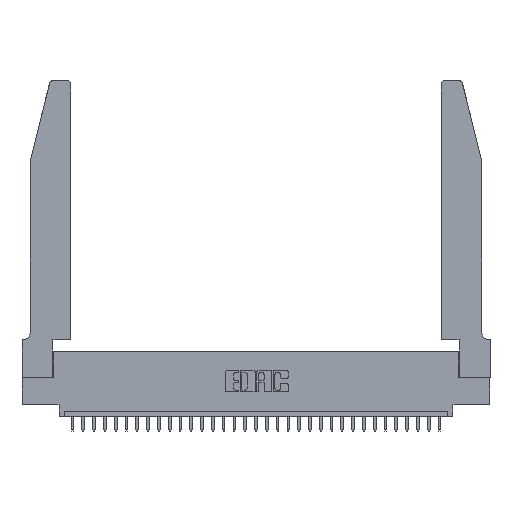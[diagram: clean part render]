
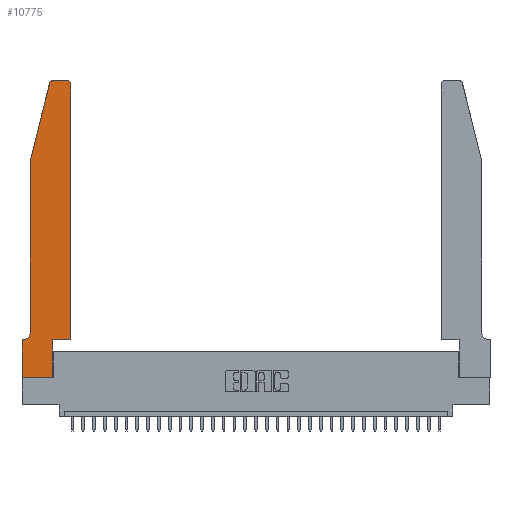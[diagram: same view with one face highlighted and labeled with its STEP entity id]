
A CAD part, top view. The second image highlights one B-rep face of the part: STEP entity #10775.
In plain terms, the highlighted planar face has unit normal (0, 0, 1).
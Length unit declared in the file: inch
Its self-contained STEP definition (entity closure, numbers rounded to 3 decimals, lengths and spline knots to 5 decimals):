
#240 = CARTESIAN_POINT ( 'NONE',  ( 0.4205, 2.72, 0.37 ) ) ;
#623 = VECTOR ( 'NONE', #9266, 39.37008 ) ;
#679 = ORIENTED_EDGE ( 'NONE', *, *, #16716, .T. ) ;
#1439 = CARTESIAN_POINT ( 'NONE',  ( 0.4505, 2.72, 0.37 ) ) ;
#1793 = CARTESIAN_POINT ( 'NONE',  ( 0.2865, 0., 0.37 ) ) ;
#2167 = LINE ( 'NONE', #10430, #25486 ) ;
#2177 = CIRCLE ( 'NONE', #19346, 0.07 ) ;
#2234 = PLANE ( 'NONE',  #19637 ) ;
#2331 = DIRECTION ( 'NONE',  ( 0., 0., 1. ) ) ;
#2535 = VECTOR ( 'NONE', #6171, 39.37008 ) ;
#2727 = DIRECTION ( 'NONE',  ( 0., 0., 1. ) ) ;
#3883 = ORIENTED_EDGE ( 'NONE', *, *, #8492, .T. ) ;
#3891 = LINE ( 'NONE', #27570, #7743 ) ;
#4243 = VERTEX_POINT ( 'NONE', #7060 ) ;
#4352 = LINE ( 'NONE', #8504, #17200 ) ;
#4415 = LINE ( 'NONE', #30306, #8326 ) ;
#4487 = CARTESIAN_POINT ( 'NONE',  ( 0.284, 2.75, 0.37 ) ) ;
#5235 = DIRECTION ( 'NONE',  ( 1., 0., 0. ) ) ;
#5300 = DIRECTION ( 'NONE',  ( 0., -1., 0. ) ) ;
#5750 = LINE ( 'NONE', #9381, #26382 ) ;
#6125 = CARTESIAN_POINT ( 'NONE',  ( 0., 0.35, 0.37 ) ) ;
#6171 = DIRECTION ( 'NONE',  ( 1., 0., 0. ) ) ;
#6735 = ORIENTED_EDGE ( 'NONE', *, *, #15269, .T. ) ;
#7060 = CARTESIAN_POINT ( 'NONE',  ( 0.4505, 0.35, 0.37 ) ) ;
#7451 = ORIENTED_EDGE ( 'NONE', *, *, #8089, .T. ) ;
#7743 = VECTOR ( 'NONE', #7985, 39.37008 ) ;
#7943 = DIRECTION ( 'NONE',  ( 0., -1., 0. ) ) ;
#7962 = VERTEX_POINT ( 'NONE', #10109 ) ;
#7985 = DIRECTION ( 'NONE',  ( -1., 0., 0. ) ) ;
#8089 = EDGE_CURVE ( 'NONE', #11727, #10027, #4352, .T. ) ;
#8212 = DIRECTION ( 'NONE',  ( 0., 0., -1. ) ) ;
#8326 = VECTOR ( 'NONE', #17617, 39.37008 ) ;
#8492 = EDGE_CURVE ( 'NONE', #19123, #4243, #9518, .T. ) ;
#8504 = CARTESIAN_POINT ( 'NONE',  ( 0.0755, 2., 0.37 ) ) ;
#9266 = DIRECTION ( 'NONE',  ( 0., 1., 0. ) ) ;
#9381 = CARTESIAN_POINT ( 'NONE',  ( 0.2865, 0.35, 0.37 ) ) ;
#9518 = LINE ( 'NONE', #30940, #2535 ) ;
#9547 = CARTESIAN_POINT ( 'NONE',  ( 0.284, 2.72, 0.37 ) ) ;
#10027 = VERTEX_POINT ( 'NONE', #22442 ) ;
#10109 = CARTESIAN_POINT ( 'NONE',  ( 0.0055, 0.35, 0.37 ) ) ;
#10288 = EDGE_LOOP ( 'NONE', ( #25359, #13772, #23497, #7451, #28519, #15678, #6735, #679, #15769, #3883, #28591, #28400 ) ) ;
#10430 = CARTESIAN_POINT ( 'NONE',  ( 0., 0., 0.37 ) ) ;
#10566 = CARTESIAN_POINT ( 'NONE',  ( 0.2865, 0.35, 0.37 ) ) ;
#10775 = ADVANCED_FACE ( 'NONE', ( #23770 ), #2234, .T. ) ;
#11593 = AXIS2_PLACEMENT_3D ( 'NONE', #240, #2727, #5235 ) ;
#11727 = VERTEX_POINT ( 'NONE', #25928 ) ;
#12066 = DIRECTION ( 'NONE',  ( 1., 0., 0. ) ) ;
#12203 = VECTOR ( 'NONE', #26372, 39.37008 ) ;
#12332 = EDGE_CURVE ( 'NONE', #15940, #11727, #15916, .T. ) ;
#13433 = EDGE_CURVE ( 'NONE', #10027, #7962, #2177, .T. ) ;
#13578 = CARTESIAN_POINT ( 'NONE',  ( 0.0055, 0.42, 0.37 ) ) ;
#13636 = CIRCLE ( 'NONE', #19750, 0.03 ) ;
#13772 = ORIENTED_EDGE ( 'NONE', *, *, #23949, .T. ) ;
#14509 = EDGE_CURVE ( 'NONE', #20005, #19123, #5750, .T. ) ;
#14687 = VERTEX_POINT ( 'NONE', #6125 ) ;
#15269 = EDGE_CURVE ( 'NONE', #14687, #28038, #2167, .T. ) ;
#15318 = CARTESIAN_POINT ( 'NONE',  ( 0.0755, 2., 0.37 ) ) ;
#15678 = ORIENTED_EDGE ( 'NONE', *, *, #24137, .T. ) ;
#15769 = ORIENTED_EDGE ( 'NONE', *, *, #14509, .T. ) ;
#15916 = LINE ( 'NONE', #15318, #21728 ) ;
#15940 = VERTEX_POINT ( 'NONE', #30138 ) ;
#16716 = EDGE_CURVE ( 'NONE', #28038, #20005, #18808, .T. ) ;
#17068 = CIRCLE ( 'NONE', #11593, 0.03 ) ;
#17200 = VECTOR ( 'NONE', #5300, 39.37008 ) ;
#17617 = DIRECTION ( 'NONE',  ( -1., 0., 0. ) ) ;
#18340 = DIRECTION ( 'NONE',  ( -1., 0., 0. ) ) ;
#18510 = LINE ( 'NONE', #26485, #623 ) ;
#18808 = LINE ( 'NONE', #31435, #12203 ) ;
#19123 = VERTEX_POINT ( 'NONE', #10566 ) ;
#19346 = AXIS2_PLACEMENT_3D ( 'NONE', #13578, #8212, #18340 ) ;
#19637 = AXIS2_PLACEMENT_3D ( 'NONE', #32131, #2331, #24763 ) ;
#19750 = AXIS2_PLACEMENT_3D ( 'NONE', #9547, #26967, #12066 ) ;
#19926 = EDGE_CURVE ( 'NONE', #26580, #24347, #17068, .T. ) ;
#20005 = VERTEX_POINT ( 'NONE', #1793 ) ;
#21728 = VECTOR ( 'NONE', #29626, 39.37008 ) ;
#21796 = EDGE_CURVE ( 'NONE', #24347, #30751, #4415, .T. ) ;
#22442 = CARTESIAN_POINT ( 'NONE',  ( 0.0755, 0.42, 0.37 ) ) ;
#22602 = DIRECTION ( 'NONE',  ( 0., 1., 0. ) ) ;
#23222 = CARTESIAN_POINT ( 'NONE',  ( 0.4205, 2.75, 0.37 ) ) ;
#23497 = ORIENTED_EDGE ( 'NONE', *, *, #12332, .T. ) ;
#23770 = FACE_OUTER_BOUND ( 'NONE', #10288, .T. ) ;
#23949 = EDGE_CURVE ( 'NONE', #30751, #15940, #13636, .T. ) ;
#24137 = EDGE_CURVE ( 'NONE', #7962, #14687, #3891, .T. ) ;
#24347 = VERTEX_POINT ( 'NONE', #23222 ) ;
#24763 = DIRECTION ( 'NONE',  ( 1., 0., 0. ) ) ;
#25359 = ORIENTED_EDGE ( 'NONE', *, *, #21796, .T. ) ;
#25486 = VECTOR ( 'NONE', #7943, 39.37008 ) ;
#25928 = CARTESIAN_POINT ( 'NONE',  ( 0.0755, 2., 0.37 ) ) ;
#26372 = DIRECTION ( 'NONE',  ( 1., 0., 0. ) ) ;
#26382 = VECTOR ( 'NONE', #22602, 39.37008 ) ;
#26485 = CARTESIAN_POINT ( 'NONE',  ( 0.4505, 0.35, 0.37 ) ) ;
#26580 = VERTEX_POINT ( 'NONE', #1439 ) ;
#26967 = DIRECTION ( 'NONE',  ( 0., 0., 1. ) ) ;
#27106 = CARTESIAN_POINT ( 'NONE',  ( 0., 0., 0.37 ) ) ;
#27570 = CARTESIAN_POINT ( 'NONE',  ( 0.0755, 0.35, 0.37 ) ) ;
#27884 = EDGE_CURVE ( 'NONE', #4243, #26580, #18510, .T. ) ;
#28038 = VERTEX_POINT ( 'NONE', #27106 ) ;
#28400 = ORIENTED_EDGE ( 'NONE', *, *, #19926, .T. ) ;
#28519 = ORIENTED_EDGE ( 'NONE', *, *, #13433, .T. ) ;
#28591 = ORIENTED_EDGE ( 'NONE', *, *, #27884, .T. ) ;
#29626 = DIRECTION ( 'NONE',  ( -0.239, -0.971, 0. ) ) ;
#30138 = CARTESIAN_POINT ( 'NONE',  ( 0.25487, 2.72718, 0.37 ) ) ;
#30306 = CARTESIAN_POINT ( 'NONE',  ( 0.2605, 2.75, 0.37 ) ) ;
#30751 = VERTEX_POINT ( 'NONE', #4487 ) ;
#30940 = CARTESIAN_POINT ( 'NONE',  ( 0.4505, 0.35, 0.37 ) ) ;
#31435 = CARTESIAN_POINT ( 'NONE',  ( 0., 0., 0.37 ) ) ;
#32131 = CARTESIAN_POINT ( 'NONE',  ( 0., 0.35, 0.37 ) ) ;
